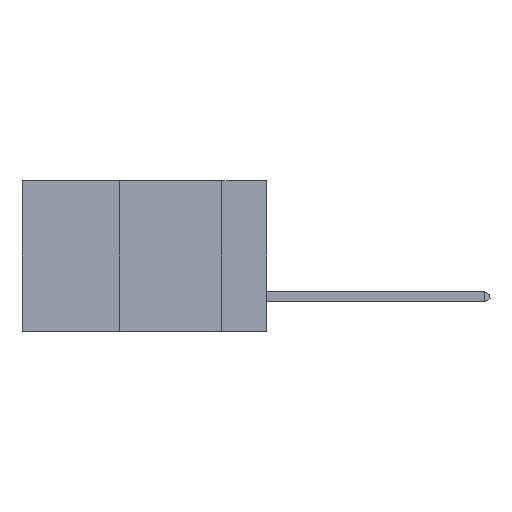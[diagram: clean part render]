
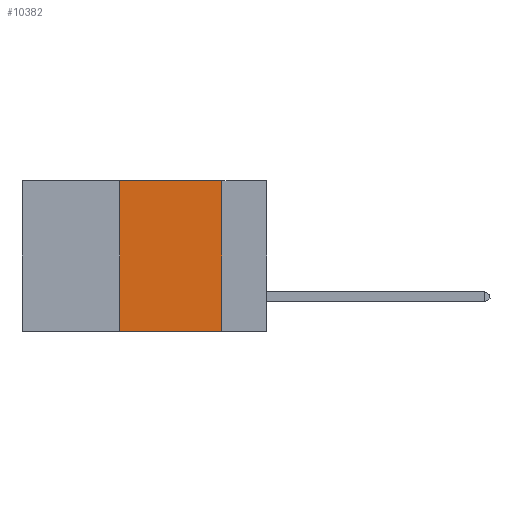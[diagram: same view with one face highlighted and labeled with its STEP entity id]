
A CAD part, left-side view. The second image highlights one B-rep face of the part: STEP entity #10382.
In plain terms, the highlighted planar face has unit normal (-1, 0, 0).
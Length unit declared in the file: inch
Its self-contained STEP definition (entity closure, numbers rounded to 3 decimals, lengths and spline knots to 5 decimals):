
#416 = AXIS2_PLACEMENT_3D ( 'NONE', #10052, #4251, #10987 ) ;
#655 = EDGE_CURVE ( 'NONE', #7300, #4331, #6168, .T. ) ;
#829 = DIRECTION ( 'NONE',  ( 0., 0., -1. ) ) ;
#1014 = VERTEX_POINT ( 'NONE', #3477 ) ;
#1139 = ORIENTED_EDGE ( 'NONE', *, *, #2156, .F. ) ;
#1193 = ORIENTED_EDGE ( 'NONE', *, *, #655, .F. ) ;
#1219 = ORIENTED_EDGE ( 'NONE', *, *, #3903, .F. ) ;
#1295 = ORIENTED_EDGE ( 'NONE', *, *, #10627, .T. ) ;
#1953 = LINE ( 'NONE', #6892, #8897 ) ;
#1968 = FACE_OUTER_BOUND ( 'NONE', #10262, .T. ) ;
#2118 = VECTOR ( 'NONE', #9595, 39.37008 ) ;
#2156 = EDGE_CURVE ( 'NONE', #4331, #1014, #1953, .T. ) ;
#2780 = CARTESIAN_POINT ( 'NONE',  ( 0., 0.36, 0. ) ) ;
#3477 = CARTESIAN_POINT ( 'NONE',  ( 0., 0.11, -0.37 ) ) ;
#3903 = EDGE_CURVE ( 'NONE', #5407, #7300, #11305, .T. ) ;
#4251 = DIRECTION ( 'NONE',  ( 1., 0., 0. ) ) ;
#4331 = VERTEX_POINT ( 'NONE', #7801 ) ;
#5407 = VERTEX_POINT ( 'NONE', #9225 ) ;
#5448 = CARTESIAN_POINT ( 'NONE',  ( 0., 0.6, 0. ) ) ;
#6168 = LINE ( 'NONE', #5448, #9071 ) ;
#6242 = VECTOR ( 'NONE', #10991, 39.37008 ) ;
#6892 = CARTESIAN_POINT ( 'NONE',  ( 0., 0.11, 0. ) ) ;
#7197 = PLANE ( 'NONE',  #416 ) ;
#7300 = VERTEX_POINT ( 'NONE', #2780 ) ;
#7801 = CARTESIAN_POINT ( 'NONE',  ( 0., 0.11, 0. ) ) ;
#8717 = CARTESIAN_POINT ( 'NONE',  ( 0., 0.6, -0.37 ) ) ;
#8897 = VECTOR ( 'NONE', #829, 39.37008 ) ;
#9071 = VECTOR ( 'NONE', #12166, 39.37008 ) ;
#9225 = CARTESIAN_POINT ( 'NONE',  ( 0., 0.36, -0.37 ) ) ;
#9335 = LINE ( 'NONE', #8717, #2118 ) ;
#9595 = DIRECTION ( 'NONE',  ( 0., -1., 0. ) ) ;
#10052 = CARTESIAN_POINT ( 'NONE',  ( 0., 0.6, 0. ) ) ;
#10262 = EDGE_LOOP ( 'NONE', ( #1139, #1193, #1219, #1295 ) ) ;
#10382 = ADVANCED_FACE ( 'NONE', ( #1968 ), #7197, .F. ) ;
#10627 = EDGE_CURVE ( 'NONE', #5407, #1014, #9335, .T. ) ;
#10977 = CARTESIAN_POINT ( 'NONE',  ( 0., 0.36, 0. ) ) ;
#10987 = DIRECTION ( 'NONE',  ( 0., 0., -1. ) ) ;
#10991 = DIRECTION ( 'NONE',  ( 0., 0., 1. ) ) ;
#11305 = LINE ( 'NONE', #10977, #6242 ) ;
#12166 = DIRECTION ( 'NONE',  ( 0., -1., 0. ) ) ;
